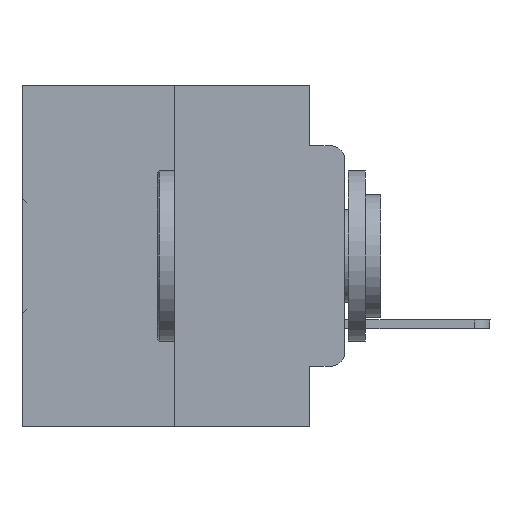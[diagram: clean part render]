
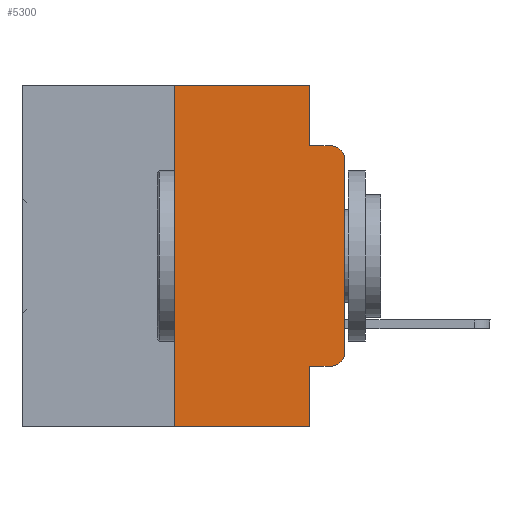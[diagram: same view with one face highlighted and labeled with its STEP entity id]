
A CAD part, left-side view. The second image highlights one B-rep face of the part: STEP entity #5300.
In plain terms, the highlighted planar face has unit normal (-1, 0, 0).
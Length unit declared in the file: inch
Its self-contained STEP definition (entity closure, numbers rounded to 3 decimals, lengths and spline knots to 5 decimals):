
#122 = VERTEX_POINT ( 'NONE', #12206 ) ;
#225 = DIRECTION ( 'NONE',  ( -1., 0., 0. ) ) ;
#633 = ORIENTED_EDGE ( 'NONE', *, *, #7724, .F. ) ;
#922 = VECTOR ( 'NONE', #32179, 39.37008 ) ;
#1160 = VERTEX_POINT ( 'NONE', #8711 ) ;
#1354 = CARTESIAN_POINT ( 'NONE',  ( 0., 0.473, -0.5 ) ) ;
#1759 = AXIS2_PLACEMENT_3D ( 'NONE', #27361, #7277, #4739 ) ;
#1958 = LINE ( 'NONE', #25253, #31183 ) ;
#2343 = DIRECTION ( 'NONE',  ( 1., 0., 0. ) ) ;
#2487 = ORIENTED_EDGE ( 'NONE', *, *, #9671, .F. ) ;
#3221 = VERTEX_POINT ( 'NONE', #3742 ) ;
#3340 = EDGE_LOOP ( 'NONE', ( #17334, #15783, #17757, #633, #29837, #2487, #17630, #21618, #28333, #27266 ) ) ;
#3742 = CARTESIAN_POINT ( 'NONE',  ( 0., 0., -0.3915 ) ) ;
#3856 = EDGE_CURVE ( 'NONE', #3221, #1160, #22101, .T. ) ;
#4739 = DIRECTION ( 'NONE',  ( 0., 0., -1. ) ) ;
#5300 = ADVANCED_FACE ( 'NONE', ( #8098 ), #15183, .F. ) ;
#5509 = AXIS2_PLACEMENT_3D ( 'NONE', #25890, #225, #12759 ) ;
#6505 = AXIS2_PLACEMENT_3D ( 'NONE', #25636, #2343, #12672 ) ;
#6914 = CARTESIAN_POINT ( 'NONE',  ( 0., 0.051, -0.0885 ) ) ;
#7277 = DIRECTION ( 'NONE',  ( -1., 0., 0. ) ) ;
#7724 = EDGE_CURVE ( 'NONE', #27158, #24244, #22129, .T. ) ;
#7868 = DIRECTION ( 'NONE',  ( 0., -1., 0. ) ) ;
#8098 = FACE_OUTER_BOUND ( 'NONE', #3340, .T. ) ;
#8507 = CARTESIAN_POINT ( 'NONE',  ( 0., 0.02, -0.4115 ) ) ;
#8711 = CARTESIAN_POINT ( 'NONE',  ( 0., 0., -0.1085 ) ) ;
#9129 = VECTOR ( 'NONE', #19246, 39.37008 ) ;
#9671 = EDGE_CURVE ( 'NONE', #13442, #29535, #26796, .T. ) ;
#9897 = CARTESIAN_POINT ( 'NONE',  ( 0., 0.473, 0. ) ) ;
#10395 = LINE ( 'NONE', #9897, #22585 ) ;
#11100 = EDGE_CURVE ( 'NONE', #24244, #122, #1958, .T. ) ;
#12206 = CARTESIAN_POINT ( 'NONE',  ( 0., 0.02, -0.0885 ) ) ;
#12672 = DIRECTION ( 'NONE',  ( 0., 0., -1. ) ) ;
#12759 = DIRECTION ( 'NONE',  ( 0., 0., -1. ) ) ;
#13018 = DIRECTION ( 'NONE',  ( 0., 0., -1. ) ) ;
#13123 = VECTOR ( 'NONE', #17363, 39.37008 ) ;
#13442 = VERTEX_POINT ( 'NONE', #19722 ) ;
#13817 = CARTESIAN_POINT ( 'NONE',  ( 0., 0.25, 0. ) ) ;
#14111 = EDGE_CURVE ( 'NONE', #13442, #20402, #21643, .T. ) ;
#14203 = CARTESIAN_POINT ( 'NONE',  ( 0., 0.051, -0.4115 ) ) ;
#14706 = VECTOR ( 'NONE', #19810, 39.37008 ) ;
#15183 = PLANE ( 'NONE',  #6505 ) ;
#15697 = CARTESIAN_POINT ( 'NONE',  ( 0., 0.051, 0. ) ) ;
#15783 = ORIENTED_EDGE ( 'NONE', *, *, #18757, .T. ) ;
#15958 = VERTEX_POINT ( 'NONE', #8507 ) ;
#16801 = VECTOR ( 'NONE', #31752, 39.37008 ) ;
#17334 = ORIENTED_EDGE ( 'NONE', *, *, #3856, .T. ) ;
#17363 = DIRECTION ( 'NONE',  ( 0., -1., 0. ) ) ;
#17630 = ORIENTED_EDGE ( 'NONE', *, *, #14111, .T. ) ;
#17757 = ORIENTED_EDGE ( 'NONE', *, *, #11100, .F. ) ;
#17919 = CIRCLE ( 'NONE', #5509, 0.02 ) ;
#18757 = EDGE_CURVE ( 'NONE', #1160, #122, #17919, .T. ) ;
#19246 = DIRECTION ( 'NONE',  ( 0., 0., 1. ) ) ;
#19722 = CARTESIAN_POINT ( 'NONE',  ( 0., 0.25, -0.5 ) ) ;
#19810 = DIRECTION ( 'NONE',  ( 0., 0., -1. ) ) ;
#19873 = EDGE_CURVE ( 'NONE', #32478, #15958, #22414, .T. ) ;
#20147 = LINE ( 'NONE', #22335, #14706 ) ;
#20402 = VERTEX_POINT ( 'NONE', #28220 ) ;
#21618 = ORIENTED_EDGE ( 'NONE', *, *, #32126, .F. ) ;
#21643 = LINE ( 'NONE', #1354, #16801 ) ;
#22101 = LINE ( 'NONE', #29864, #9129 ) ;
#22129 = LINE ( 'NONE', #28517, #23321 ) ;
#22232 = DIRECTION ( 'NONE',  ( 0., -1., 0. ) ) ;
#22335 = CARTESIAN_POINT ( 'NONE',  ( 0., 0.051, 0. ) ) ;
#22414 = LINE ( 'NONE', #29664, #13123 ) ;
#22585 = VECTOR ( 'NONE', #7868, 39.37008 ) ;
#23321 = VECTOR ( 'NONE', #13018, 39.37008 ) ;
#24244 = VERTEX_POINT ( 'NONE', #6914 ) ;
#25253 = CARTESIAN_POINT ( 'NONE',  ( 0., 0.051, -0.0885 ) ) ;
#25636 = CARTESIAN_POINT ( 'NONE',  ( 0., 0.473, 0. ) ) ;
#25890 = CARTESIAN_POINT ( 'NONE',  ( 0., 0.02, -0.1085 ) ) ;
#26796 = LINE ( 'NONE', #13817, #922 ) ;
#27158 = VERTEX_POINT ( 'NONE', #15697 ) ;
#27266 = ORIENTED_EDGE ( 'NONE', *, *, #32614, .T. ) ;
#27361 = CARTESIAN_POINT ( 'NONE',  ( 0., 0.02, -0.3915 ) ) ;
#28220 = CARTESIAN_POINT ( 'NONE',  ( 0., 0.051, -0.5 ) ) ;
#28333 = ORIENTED_EDGE ( 'NONE', *, *, #19873, .T. ) ;
#28517 = CARTESIAN_POINT ( 'NONE',  ( 0., 0.051, 0. ) ) ;
#29266 = CIRCLE ( 'NONE', #1759, 0.02 ) ;
#29331 = EDGE_CURVE ( 'NONE', #29535, #27158, #10395, .T. ) ;
#29535 = VERTEX_POINT ( 'NONE', #31961 ) ;
#29664 = CARTESIAN_POINT ( 'NONE',  ( 0., 0.051, -0.4115 ) ) ;
#29837 = ORIENTED_EDGE ( 'NONE', *, *, #29331, .F. ) ;
#29864 = CARTESIAN_POINT ( 'NONE',  ( 0., 0., 0. ) ) ;
#31183 = VECTOR ( 'NONE', #22232, 39.37008 ) ;
#31752 = DIRECTION ( 'NONE',  ( 0., -1., 0. ) ) ;
#31961 = CARTESIAN_POINT ( 'NONE',  ( 0., 0.25, 0. ) ) ;
#32126 = EDGE_CURVE ( 'NONE', #32478, #20402, #20147, .T. ) ;
#32179 = DIRECTION ( 'NONE',  ( 0., 0., 1. ) ) ;
#32478 = VERTEX_POINT ( 'NONE', #14203 ) ;
#32614 = EDGE_CURVE ( 'NONE', #15958, #3221, #29266, .T. ) ;
